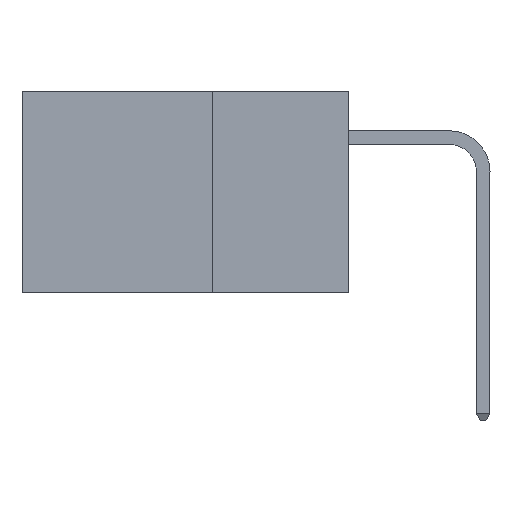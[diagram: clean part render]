
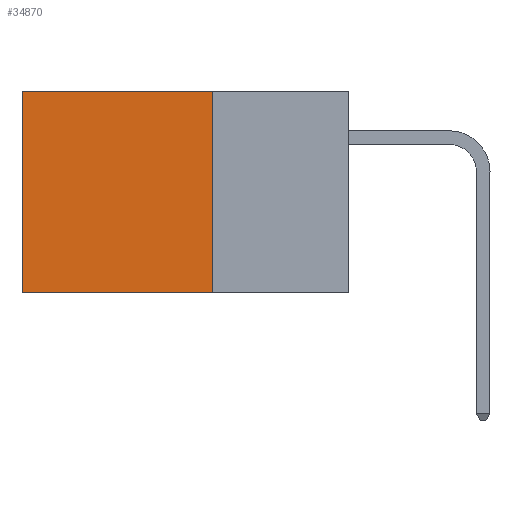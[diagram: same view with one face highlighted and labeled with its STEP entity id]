
A CAD part, left-side view. The second image highlights one B-rep face of the part: STEP entity #34870.
In plain terms, the highlighted planar face has unit normal (-1, 0, 0).
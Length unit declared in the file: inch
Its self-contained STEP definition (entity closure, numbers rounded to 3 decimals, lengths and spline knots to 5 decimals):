
#154 = VECTOR ( 'NONE', #20469, 39.37008 ) ;
#255 = ORIENTED_EDGE ( 'NONE', *, *, #26366, .T. ) ;
#943 = EDGE_LOOP ( 'NONE', ( #255, #14902, #31697, #25704 ) ) ;
#2748 = LINE ( 'NONE', #18058, #23427 ) ;
#4417 = DIRECTION ( 'NONE',  ( 1., 0., 0. ) ) ;
#5477 = EDGE_CURVE ( 'NONE', #26526, #34605, #15426, .T. ) ;
#5559 = CARTESIAN_POINT ( 'NONE',  ( 0.2875, 0.6, -0.37 ) ) ;
#5974 = VECTOR ( 'NONE', #16801, 39.37008 ) ;
#6198 = LINE ( 'NONE', #25252, #26808 ) ;
#6553 = FACE_OUTER_BOUND ( 'NONE', #943, .T. ) ;
#6881 = CARTESIAN_POINT ( 'NONE',  ( 0.2875, 0.25, -0.37 ) ) ;
#7201 = PLANE ( 'NONE',  #15994 ) ;
#9677 = DIRECTION ( 'NONE',  ( 0., 1., 0. ) ) ;
#11996 = VERTEX_POINT ( 'NONE', #23424 ) ;
#12805 = EDGE_CURVE ( 'NONE', #28566, #26526, #13527, .T. ) ;
#13527 = LINE ( 'NONE', #35713, #5974 ) ;
#14206 = DIRECTION ( 'NONE',  ( 0., 0., -1. ) ) ;
#14902 = ORIENTED_EDGE ( 'NONE', *, *, #5477, .F. ) ;
#15426 = LINE ( 'NONE', #23089, #154 ) ;
#15994 = AXIS2_PLACEMENT_3D ( 'NONE', #34969, #4417, #24056 ) ;
#16236 = CARTESIAN_POINT ( 'NONE',  ( 0.2875, 0.25, 0. ) ) ;
#16801 = DIRECTION ( 'NONE',  ( 0., 0., -1. ) ) ;
#18058 = CARTESIAN_POINT ( 'NONE',  ( 0.2875, 0.25, 0. ) ) ;
#20469 = DIRECTION ( 'NONE',  ( 0., 1., 0. ) ) ;
#23089 = CARTESIAN_POINT ( 'NONE',  ( 0.2875, 0.25, -0.37 ) ) ;
#23424 = CARTESIAN_POINT ( 'NONE',  ( 0.2875, 0.6, 0. ) ) ;
#23427 = VECTOR ( 'NONE', #9677, 39.37008 ) ;
#24056 = DIRECTION ( 'NONE',  ( 0., 0., -1. ) ) ;
#25252 = CARTESIAN_POINT ( 'NONE',  ( 0.2875, 0.6, 0. ) ) ;
#25704 = ORIENTED_EDGE ( 'NONE', *, *, #31523, .T. ) ;
#26366 = EDGE_CURVE ( 'NONE', #11996, #34605, #6198, .T. ) ;
#26526 = VERTEX_POINT ( 'NONE', #6881 ) ;
#26808 = VECTOR ( 'NONE', #14206, 39.37008 ) ;
#28566 = VERTEX_POINT ( 'NONE', #16236 ) ;
#31523 = EDGE_CURVE ( 'NONE', #28566, #11996, #2748, .T. ) ;
#31697 = ORIENTED_EDGE ( 'NONE', *, *, #12805, .F. ) ;
#34605 = VERTEX_POINT ( 'NONE', #5559 ) ;
#34870 = ADVANCED_FACE ( 'NONE', ( #6553 ), #7201, .F. ) ;
#34969 = CARTESIAN_POINT ( 'NONE',  ( 0.2875, 0.25, 0. ) ) ;
#35713 = CARTESIAN_POINT ( 'NONE',  ( 0.2875, 0.25, 0. ) ) ;
